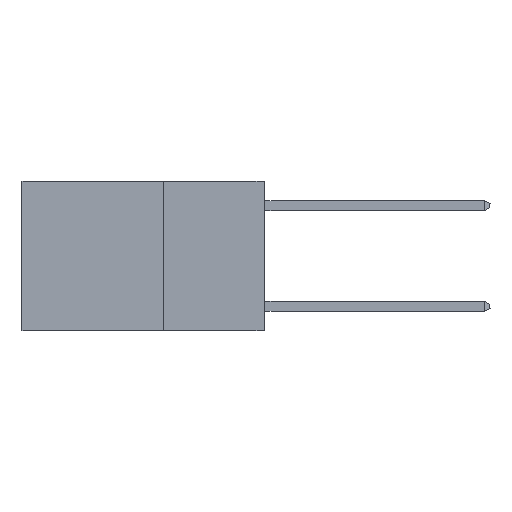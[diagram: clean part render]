
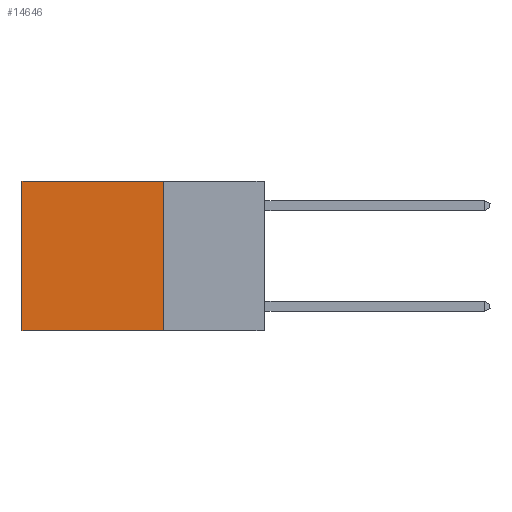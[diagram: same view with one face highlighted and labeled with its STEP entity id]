
A CAD part, left-side view. The second image highlights one B-rep face of the part: STEP entity #14646.
In plain terms, the highlighted planar face has unit normal (-1, 0, 0).
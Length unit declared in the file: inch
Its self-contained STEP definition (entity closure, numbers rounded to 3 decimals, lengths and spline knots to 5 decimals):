
#547 = EDGE_CURVE ( 'NONE', #8864, #6554, #10007, .T. ) ;
#660 = CARTESIAN_POINT ( 'NONE',  ( 0.2625, 0.25, -0.37 ) ) ;
#1061 = ORIENTED_EDGE ( 'NONE', *, *, #547, .F. ) ;
#1134 = EDGE_LOOP ( 'NONE', ( #1809, #1061, #9994, #3444 ) ) ;
#1293 = CARTESIAN_POINT ( 'NONE',  ( 0.2625, 0.25, 0. ) ) ;
#1391 = CARTESIAN_POINT ( 'NONE',  ( 0.2625, 0.6, 0. ) ) ;
#1741 = DIRECTION ( 'NONE',  ( 0., 0., -1. ) ) ;
#1809 = ORIENTED_EDGE ( 'NONE', *, *, #4126, .T. ) ;
#2474 = VECTOR ( 'NONE', #12458, 39.37008 ) ;
#2835 = LINE ( 'NONE', #14840, #2474 ) ;
#3444 = ORIENTED_EDGE ( 'NONE', *, *, #12917, .T. ) ;
#3686 = PLANE ( 'NONE',  #3984 ) ;
#3909 = DIRECTION ( 'NONE',  ( 1., 0., 0. ) ) ;
#3984 = AXIS2_PLACEMENT_3D ( 'NONE', #1293, #3909, #9776 ) ;
#4126 = EDGE_CURVE ( 'NONE', #4779, #6554, #6702, .T. ) ;
#4779 = VERTEX_POINT ( 'NONE', #1391 ) ;
#5145 = DIRECTION ( 'NONE',  ( 0., 1., 0. ) ) ;
#5370 = CARTESIAN_POINT ( 'NONE',  ( 0.2625, 0.6, 0. ) ) ;
#5568 = VERTEX_POINT ( 'NONE', #13824 ) ;
#6554 = VERTEX_POINT ( 'NONE', #12197 ) ;
#6702 = LINE ( 'NONE', #5370, #8539 ) ;
#7913 = LINE ( 'NONE', #14975, #12251 ) ;
#8539 = VECTOR ( 'NONE', #1741, 39.37008 ) ;
#8864 = VERTEX_POINT ( 'NONE', #10987 ) ;
#9776 = DIRECTION ( 'NONE',  ( 0., 0., -1. ) ) ;
#9994 = ORIENTED_EDGE ( 'NONE', *, *, #11270, .F. ) ;
#10007 = LINE ( 'NONE', #660, #13924 ) ;
#10342 = DIRECTION ( 'NONE',  ( 0., 1., 0. ) ) ;
#10987 = CARTESIAN_POINT ( 'NONE',  ( 0.2625, 0.25, -0.37 ) ) ;
#11270 = EDGE_CURVE ( 'NONE', #5568, #8864, #2835, .T. ) ;
#12197 = CARTESIAN_POINT ( 'NONE',  ( 0.2625, 0.6, -0.37 ) ) ;
#12251 = VECTOR ( 'NONE', #10342, 39.37008 ) ;
#12458 = DIRECTION ( 'NONE',  ( 0., 0., -1. ) ) ;
#12917 = EDGE_CURVE ( 'NONE', #5568, #4779, #7913, .T. ) ;
#13824 = CARTESIAN_POINT ( 'NONE',  ( 0.2625, 0.25, 0. ) ) ;
#13924 = VECTOR ( 'NONE', #5145, 39.37008 ) ;
#14354 = FACE_OUTER_BOUND ( 'NONE', #1134, .T. ) ;
#14646 = ADVANCED_FACE ( 'NONE', ( #14354 ), #3686, .F. ) ;
#14840 = CARTESIAN_POINT ( 'NONE',  ( 0.2625, 0.25, 0. ) ) ;
#14975 = CARTESIAN_POINT ( 'NONE',  ( 0.2625, 0.25, 0. ) ) ;
